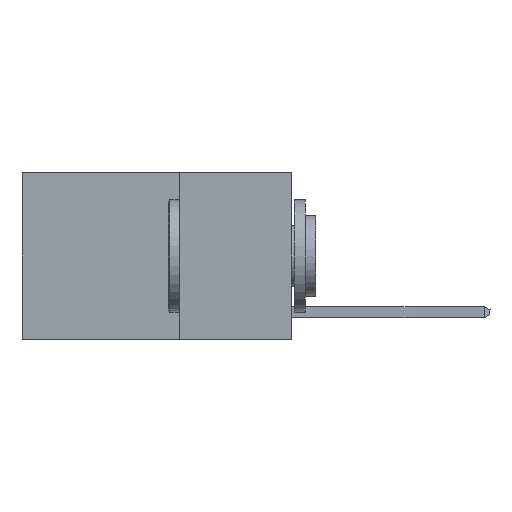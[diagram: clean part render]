
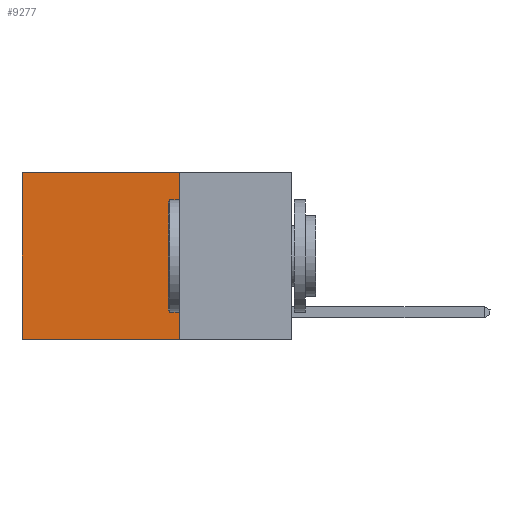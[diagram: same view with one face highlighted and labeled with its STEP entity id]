
A CAD part, left-side view. The second image highlights one B-rep face of the part: STEP entity #9277.
In plain terms, the highlighted planar face has unit normal (-1, 0, 0).
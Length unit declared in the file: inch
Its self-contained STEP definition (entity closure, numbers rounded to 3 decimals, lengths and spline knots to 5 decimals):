
#692 = CARTESIAN_POINT ( 'NONE',  ( 0.2625, 0.6, 0. ) ) ;
#829 = CARTESIAN_POINT ( 'NONE',  ( 0.2625, 0.25, 0. ) ) ;
#2588 = ORIENTED_EDGE ( 'NONE', *, *, #17336, .F. ) ;
#2972 = CARTESIAN_POINT ( 'NONE',  ( 0.2625, 0.25, 0. ) ) ;
#3227 = VERTEX_POINT ( 'NONE', #13970 ) ;
#4218 = ORIENTED_EDGE ( 'NONE', *, *, #20622, .F. ) ;
#5658 = CARTESIAN_POINT ( 'NONE',  ( 0.2625, 0.25, -0.37 ) ) ;
#6276 = DIRECTION ( 'NONE',  ( 0., 0., -1. ) ) ;
#6650 = DIRECTION ( 'NONE',  ( 0., 1., 0. ) ) ;
#7693 = AXIS2_PLACEMENT_3D ( 'NONE', #10535, #12716, #10618 ) ;
#8069 = VECTOR ( 'NONE', #11370, 39.37008 ) ;
#9277 = ADVANCED_FACE ( 'NONE', ( #20211 ), #18359, .F. ) ;
#9922 = VERTEX_POINT ( 'NONE', #692 ) ;
#10535 = CARTESIAN_POINT ( 'NONE',  ( 0.2625, 0.25, 0. ) ) ;
#10618 = DIRECTION ( 'NONE',  ( 0., 0., -1. ) ) ;
#11370 = DIRECTION ( 'NONE',  ( 0., 1., 0. ) ) ;
#11875 = VECTOR ( 'NONE', #16405, 39.37008 ) ;
#12080 = ORIENTED_EDGE ( 'NONE', *, *, #19774, .T. ) ;
#12716 = DIRECTION ( 'NONE',  ( 1., 0., 0. ) ) ;
#13156 = LINE ( 'NONE', #23125, #8069 ) ;
#13970 = CARTESIAN_POINT ( 'NONE',  ( 0.2625, 0.6, -0.37 ) ) ;
#14050 = CARTESIAN_POINT ( 'NONE',  ( 0.2625, 0.6, 0. ) ) ;
#14419 = VECTOR ( 'NONE', #6276, 39.37008 ) ;
#14910 = VECTOR ( 'NONE', #6650, 39.37008 ) ;
#15799 = LINE ( 'NONE', #829, #14910 ) ;
#16156 = VERTEX_POINT ( 'NONE', #19839 ) ;
#16405 = DIRECTION ( 'NONE',  ( 0., 0., -1. ) ) ;
#16529 = EDGE_LOOP ( 'NONE', ( #12080, #4218, #2588, #20383 ) ) ;
#16980 = LINE ( 'NONE', #2972, #11875 ) ;
#17336 = EDGE_CURVE ( 'NONE', #16156, #17481, #16980, .T. ) ;
#17481 = VERTEX_POINT ( 'NONE', #5658 ) ;
#18359 = PLANE ( 'NONE',  #7693 ) ;
#19774 = EDGE_CURVE ( 'NONE', #9922, #3227, #24632, .T. ) ;
#19839 = CARTESIAN_POINT ( 'NONE',  ( 0.2625, 0.25, 0. ) ) ;
#20211 = FACE_OUTER_BOUND ( 'NONE', #16529, .T. ) ;
#20383 = ORIENTED_EDGE ( 'NONE', *, *, #22724, .T. ) ;
#20622 = EDGE_CURVE ( 'NONE', #17481, #3227, #13156, .T. ) ;
#22724 = EDGE_CURVE ( 'NONE', #16156, #9922, #15799, .T. ) ;
#23125 = CARTESIAN_POINT ( 'NONE',  ( 0.2625, 0.25, -0.37 ) ) ;
#24632 = LINE ( 'NONE', #14050, #14419 ) ;
